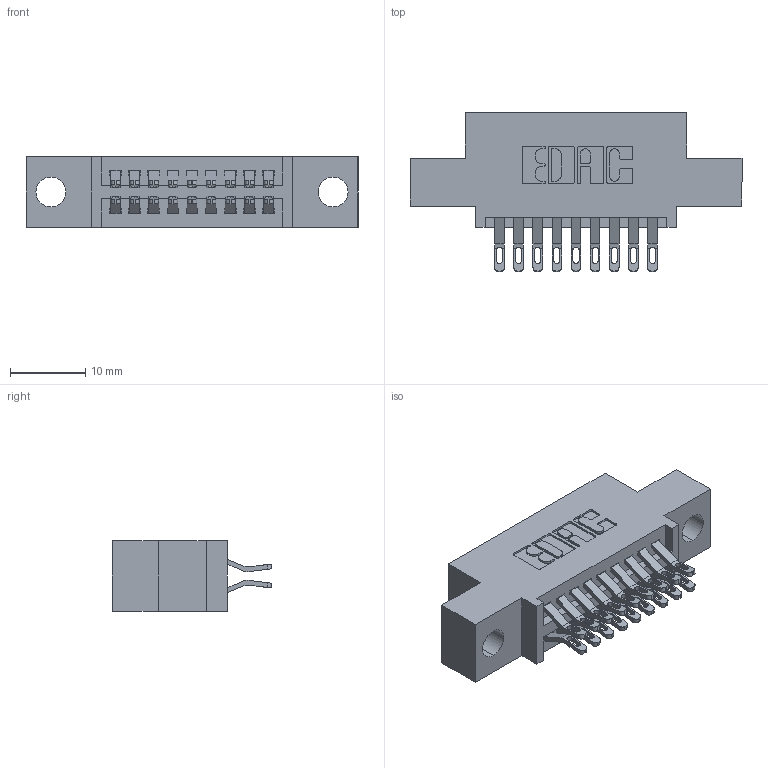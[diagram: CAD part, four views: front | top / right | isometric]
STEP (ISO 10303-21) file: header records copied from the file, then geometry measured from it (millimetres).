
FILE_DESCRIPTION (( 'STEP AP203' ), '1' );
FILE_NAME ('345-018-555-504.STEP', '2021-05-19T16:41:29', ( '' ), ( '' ), 'SwSTEP 2.0', 'SolidWorks 2020', '' );
FILE_SCHEMA (( 'CONFIG_CONTROL_DESIGN' ));
Length unit declared in the file: inch
Products named in the file (3): 345 Part_0.110 Offset - 0.156 Dia-TI; 345-018-555-504; 345-292-001_555 Tail
Assembly tree (19 placements, depth 2):
  345-018-555-504
    345 Part_0.110 Offset - 0.156 Dia-TI
    345-292-001_555 Tail  x18
Bounding box: 44.07 x 21.13 x 9.4 mm (x, y, z)
Volume: 3847.5 mm3; surface area: 5174.1 mm2
Topology: 19 solids, 19 shells, 1152 faces, 3575 edges, 2382 vertices
Faces by surface type: plane 656, cylinder 496
Entity records: 12381 total; most frequent: CARTESIAN_POINT 2148, ORIENTED_EDGE 2050, DIRECTION 1901, EDGE_CURVE 1025, VECTOR 837, LINE 837, VERTEX_POINT 682, AXIS2_PLACEMENT_3D 532
